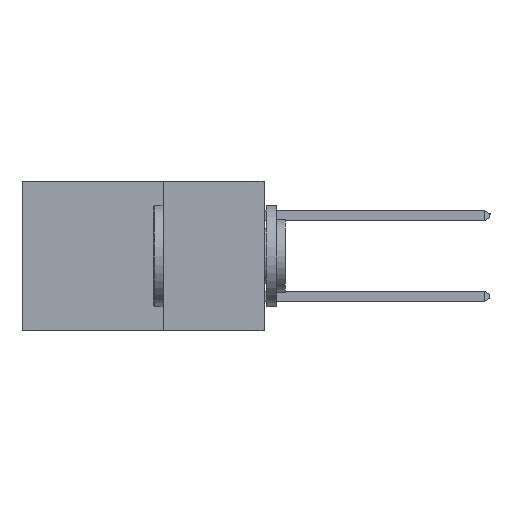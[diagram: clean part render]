
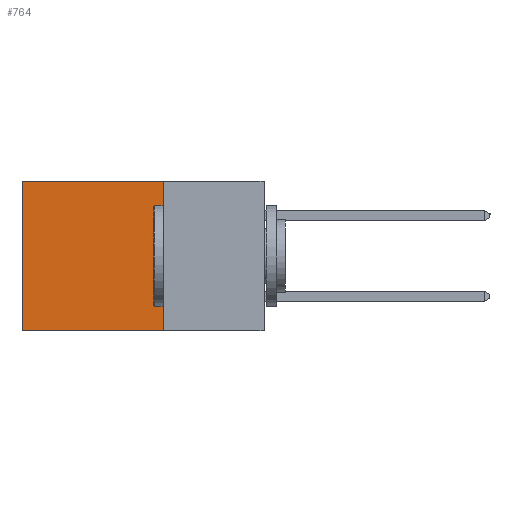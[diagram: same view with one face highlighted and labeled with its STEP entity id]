
A CAD part, left-side view. The second image highlights one B-rep face of the part: STEP entity #764.
In plain terms, the highlighted planar face has unit normal (-1, 0, 0).
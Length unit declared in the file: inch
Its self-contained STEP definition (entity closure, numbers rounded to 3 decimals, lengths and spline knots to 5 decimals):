
#83 = VECTOR ( 'NONE', #10617, 39.37008 ) ;
#764 = ADVANCED_FACE ( 'NONE', ( #17642 ), #10959, .F. ) ;
#1747 = LINE ( 'NONE', #21611, #5288 ) ;
#3515 = LINE ( 'NONE', #18001, #17284 ) ;
#4782 = ORIENTED_EDGE ( 'NONE', *, *, #5880, .T. ) ;
#5147 = VERTEX_POINT ( 'NONE', #18413 ) ;
#5288 = VECTOR ( 'NONE', #10852, 39.37008 ) ;
#5674 = DIRECTION ( 'NONE',  ( 0., 1., 0. ) ) ;
#5709 = ORIENTED_EDGE ( 'NONE', *, *, #6873, .T. ) ;
#5880 = EDGE_CURVE ( 'NONE', #5147, #22370, #3515, .T. ) ;
#6873 = EDGE_CURVE ( 'NONE', #10322, #5147, #14536, .T. ) ;
#7269 = EDGE_LOOP ( 'NONE', ( #4782, #14287, #16800, #5709 ) ) ;
#8967 = CARTESIAN_POINT ( 'NONE',  ( 0.2615, 0.6, -0.37 ) ) ;
#8982 = CARTESIAN_POINT ( 'NONE',  ( 0.2615, 0.25, 0. ) ) ;
#10155 = AXIS2_PLACEMENT_3D ( 'NONE', #19619, #21387, #16228 ) ;
#10322 = VERTEX_POINT ( 'NONE', #8982 ) ;
#10380 = EDGE_CURVE ( 'NONE', #10322, #21238, #16208, .T. ) ;
#10617 = DIRECTION ( 'NONE',  ( 0., 0., -1. ) ) ;
#10824 = CARTESIAN_POINT ( 'NONE',  ( 0.2615, 0.25, -0.37 ) ) ;
#10852 = DIRECTION ( 'NONE',  ( 0., 1., 0. ) ) ;
#10959 = PLANE ( 'NONE',  #10155 ) ;
#13021 = VECTOR ( 'NONE', #5674, 39.37008 ) ;
#13584 = CARTESIAN_POINT ( 'NONE',  ( 0.2615, 0.25, -0.37 ) ) ;
#13989 = EDGE_CURVE ( 'NONE', #21238, #22370, #1747, .T. ) ;
#14257 = DIRECTION ( 'NONE',  ( 0., 0., -1. ) ) ;
#14287 = ORIENTED_EDGE ( 'NONE', *, *, #13989, .F. ) ;
#14536 = LINE ( 'NONE', #21675, #13021 ) ;
#16208 = LINE ( 'NONE', #10824, #83 ) ;
#16228 = DIRECTION ( 'NONE',  ( 0., 0., -1. ) ) ;
#16800 = ORIENTED_EDGE ( 'NONE', *, *, #10380, .F. ) ;
#17284 = VECTOR ( 'NONE', #14257, 39.37008 ) ;
#17642 = FACE_OUTER_BOUND ( 'NONE', #7269, .T. ) ;
#18001 = CARTESIAN_POINT ( 'NONE',  ( 0.2615, 0.6, -0.37 ) ) ;
#18413 = CARTESIAN_POINT ( 'NONE',  ( 0.2615, 0.6, 0. ) ) ;
#19619 = CARTESIAN_POINT ( 'NONE',  ( 0.2615, 0.25, -0.37 ) ) ;
#21238 = VERTEX_POINT ( 'NONE', #13584 ) ;
#21387 = DIRECTION ( 'NONE',  ( 1., 0., 0. ) ) ;
#21611 = CARTESIAN_POINT ( 'NONE',  ( 0.2615, 0.25, -0.37 ) ) ;
#21675 = CARTESIAN_POINT ( 'NONE',  ( 0.2615, 0.25, 0. ) ) ;
#22370 = VERTEX_POINT ( 'NONE', #8967 ) ;
